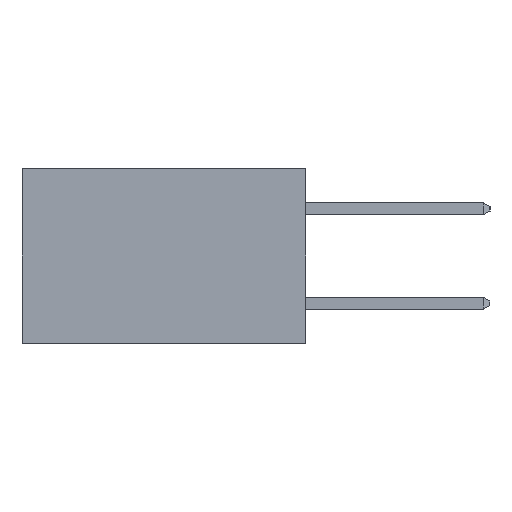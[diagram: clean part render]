
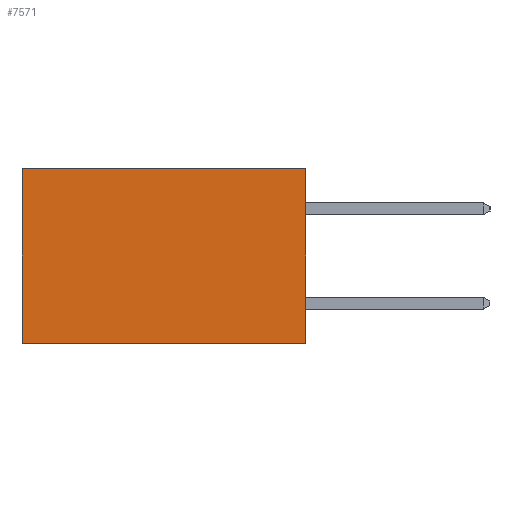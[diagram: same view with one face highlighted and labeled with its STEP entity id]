
A CAD part, left-side view. The second image highlights one B-rep face of the part: STEP entity #7571.
In plain terms, the highlighted planar face has unit normal (-1, 0, 0).
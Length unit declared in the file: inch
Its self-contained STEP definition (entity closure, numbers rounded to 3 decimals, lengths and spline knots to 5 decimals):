
#963 = LINE ( 'NONE', #8717, #7176 ) ;
#1039 = VERTEX_POINT ( 'NONE', #13304 ) ;
#1149 = FACE_OUTER_BOUND ( 'NONE', #13554, .T. ) ;
#1343 = EDGE_CURVE ( 'NONE', #14717, #9103, #2760, .T. ) ;
#1876 = DIRECTION ( 'NONE',  ( 0., 0., -1. ) ) ;
#2423 = CARTESIAN_POINT ( 'NONE',  ( 0.298, 0., 0. ) ) ;
#2760 = LINE ( 'NONE', #10884, #15643 ) ;
#4210 = ORIENTED_EDGE ( 'NONE', *, *, #12856, .T. ) ;
#5933 = ORIENTED_EDGE ( 'NONE', *, *, #1343, .T. ) ;
#6294 = EDGE_CURVE ( 'NONE', #1039, #13174, #963, .T. ) ;
#6792 = PLANE ( 'NONE',  #7266 ) ;
#7176 = VECTOR ( 'NONE', #12514, 39.37008 ) ;
#7266 = AXIS2_PLACEMENT_3D ( 'NONE', #8066, #9363, #1876 ) ;
#7571 = ADVANCED_FACE ( 'NONE', ( #1149 ), #6792, .F. ) ;
#7617 = CARTESIAN_POINT ( 'NONE',  ( 0.298, 0.6, -0.37 ) ) ;
#7667 = VECTOR ( 'NONE', #8641, 39.37008 ) ;
#8066 = CARTESIAN_POINT ( 'NONE',  ( 0.298, 0., 0. ) ) ;
#8641 = DIRECTION ( 'NONE',  ( 0., 0., -1. ) ) ;
#8717 = CARTESIAN_POINT ( 'NONE',  ( 0.298, 0., -0.37 ) ) ;
#9103 = VERTEX_POINT ( 'NONE', #11238 ) ;
#9315 = ORIENTED_EDGE ( 'NONE', *, *, #6294, .F. ) ;
#9363 = DIRECTION ( 'NONE',  ( 1., 0., 0. ) ) ;
#9391 = DIRECTION ( 'NONE',  ( 0., 1., 0. ) ) ;
#10787 = CARTESIAN_POINT ( 'NONE',  ( 0.298, 0., 0. ) ) ;
#10884 = CARTESIAN_POINT ( 'NONE',  ( 0.298, 0., 0. ) ) ;
#10888 = CARTESIAN_POINT ( 'NONE',  ( 0.298, 0.6, 0. ) ) ;
#11238 = CARTESIAN_POINT ( 'NONE',  ( 0.298, 0.6, 0. ) ) ;
#11422 = LINE ( 'NONE', #2423, #7667 ) ;
#12149 = DIRECTION ( 'NONE',  ( 0., 0., -1. ) ) ;
#12484 = VECTOR ( 'NONE', #12149, 39.37008 ) ;
#12514 = DIRECTION ( 'NONE',  ( 0., 1., 0. ) ) ;
#12657 = ORIENTED_EDGE ( 'NONE', *, *, #16114, .F. ) ;
#12856 = EDGE_CURVE ( 'NONE', #9103, #13174, #15755, .T. ) ;
#13174 = VERTEX_POINT ( 'NONE', #7617 ) ;
#13304 = CARTESIAN_POINT ( 'NONE',  ( 0.298, 0., -0.37 ) ) ;
#13554 = EDGE_LOOP ( 'NONE', ( #4210, #9315, #12657, #5933 ) ) ;
#14717 = VERTEX_POINT ( 'NONE', #10787 ) ;
#15643 = VECTOR ( 'NONE', #9391, 39.37008 ) ;
#15755 = LINE ( 'NONE', #10888, #12484 ) ;
#16114 = EDGE_CURVE ( 'NONE', #14717, #1039, #11422, .T. ) ;
